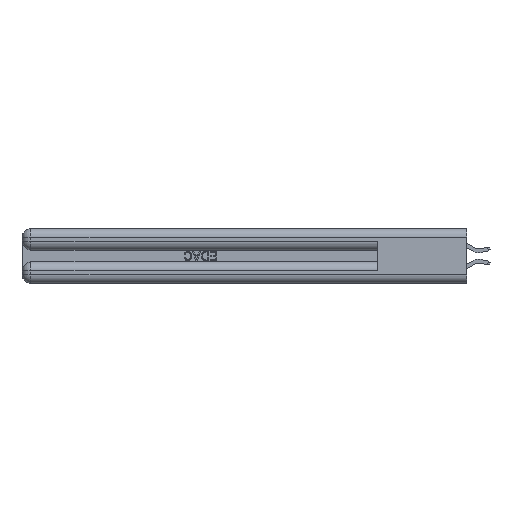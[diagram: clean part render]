
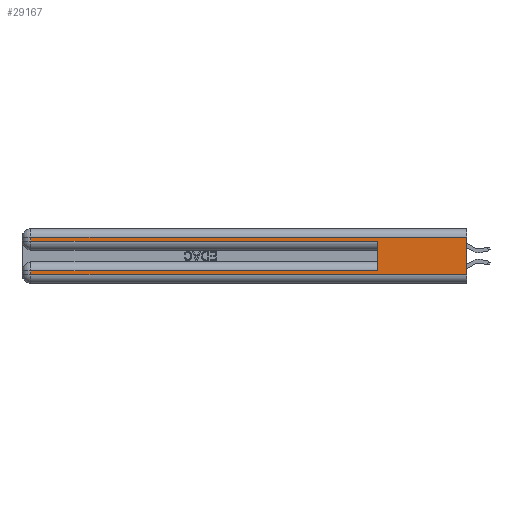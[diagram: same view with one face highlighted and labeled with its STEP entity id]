
A CAD part, left-side view. The second image highlights one B-rep face of the part: STEP entity #29167.
In plain terms, the highlighted planar face has unit normal (-1, 0, 0).
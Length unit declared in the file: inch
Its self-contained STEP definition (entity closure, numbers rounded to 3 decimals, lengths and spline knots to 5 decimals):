
#72 = CARTESIAN_POINT ( 'NONE',  ( 0., 0.6, 0.285 ) ) ;
#311 = EDGE_CURVE ( 'NONE', #539, #42509, #31341, .T. ) ;
#539 = VERTEX_POINT ( 'NONE', #27123 ) ;
#3515 = VERTEX_POINT ( 'NONE', #72 ) ;
#4661 = EDGE_CURVE ( 'NONE', #33282, #26031, #31007, .T. ) ;
#6247 = VERTEX_POINT ( 'NONE', #28322 ) ;
#6253 = CARTESIAN_POINT ( 'NONE',  ( 0., 0., 0.31 ) ) ;
#6600 = DIRECTION ( 'NONE',  ( 0., -1., 0. ) ) ;
#6920 = CARTESIAN_POINT ( 'NONE',  ( 0., 2.94, 0.285 ) ) ;
#7168 = ORIENTED_EDGE ( 'NONE', *, *, #311, .F. ) ;
#7199 = PLANE ( 'NONE',  #31934 ) ;
#7261 = ORIENTED_EDGE ( 'NONE', *, *, #28585, .T. ) ;
#7619 = VECTOR ( 'NONE', #19460, 39.37008 ) ;
#10107 = DIRECTION ( 'NONE',  ( 1., 0., 0. ) ) ;
#10196 = DIRECTION ( 'NONE',  ( 0., 0., -1. ) ) ;
#10818 = CARTESIAN_POINT ( 'NONE',  ( 0., 0.6, 0.145 ) ) ;
#11771 = CARTESIAN_POINT ( 'NONE',  ( 0., 2.94, 0.06 ) ) ;
#12688 = CARTESIAN_POINT ( 'NONE',  ( 0., 0., 0.285 ) ) ;
#13063 = DIRECTION ( 'NONE',  ( 0., 1., 0. ) ) ;
#13878 = EDGE_CURVE ( 'NONE', #539, #33282, #35832, .T. ) ;
#14677 = DIRECTION ( 'NONE',  ( 0., 0., -1. ) ) ;
#15259 = VERTEX_POINT ( 'NONE', #18500 ) ;
#15513 = VERTEX_POINT ( 'NONE', #11771 ) ;
#16956 = ORIENTED_EDGE ( 'NONE', *, *, #28069, .F. ) ;
#18350 = VECTOR ( 'NONE', #36685, 39.37008 ) ;
#18500 = CARTESIAN_POINT ( 'NONE',  ( 0., 2.94, 0.085 ) ) ;
#19460 = DIRECTION ( 'NONE',  ( 0., -1., 0. ) ) ;
#19883 = ORIENTED_EDGE ( 'NONE', *, *, #37157, .T. ) ;
#20031 = ORIENTED_EDGE ( 'NONE', *, *, #35923, .T. ) ;
#21222 = CARTESIAN_POINT ( 'NONE',  ( 0., 0., 0.06 ) ) ;
#22033 = ORIENTED_EDGE ( 'NONE', *, *, #35537, .T. ) ;
#22641 = CARTESIAN_POINT ( 'NONE',  ( 0., 2.94, 0.31 ) ) ;
#22929 = FACE_OUTER_BOUND ( 'NONE', #34871, .T. ) ;
#23273 = DIRECTION ( 'NONE',  ( 0., 0., -1. ) ) ;
#24306 = VECTOR ( 'NONE', #10196, 39.37008 ) ;
#26031 = VERTEX_POINT ( 'NONE', #6920 ) ;
#26415 = CARTESIAN_POINT ( 'NONE',  ( 0., 0., 0.06 ) ) ;
#27123 = CARTESIAN_POINT ( 'NONE',  ( 0., 0., 0.31 ) ) ;
#28069 = EDGE_CURVE ( 'NONE', #6247, #3515, #40621, .T. ) ;
#28322 = CARTESIAN_POINT ( 'NONE',  ( 0., 0.6, 0.085 ) ) ;
#28585 = EDGE_CURVE ( 'NONE', #15513, #42509, #28679, .T. ) ;
#28679 = LINE ( 'NONE', #26415, #36419 ) ;
#28843 = DIRECTION ( 'NONE',  ( 0., 1., 0. ) ) ;
#29167 = ADVANCED_FACE ( 'NONE', ( #22929 ), #7199, .F. ) ;
#30457 = VECTOR ( 'NONE', #13063, 39.37008 ) ;
#31007 = LINE ( 'NONE', #40410, #24306 ) ;
#31341 = LINE ( 'NONE', #39829, #42304 ) ;
#31934 = AXIS2_PLACEMENT_3D ( 'NONE', #36413, #10107, #23273 ) ;
#33036 = LINE ( 'NONE', #36187, #30457 ) ;
#33282 = VERTEX_POINT ( 'NONE', #22641 ) ;
#34259 = DIRECTION ( 'NONE',  ( 0., 0., -1. ) ) ;
#34871 = EDGE_LOOP ( 'NONE', ( #7168, #38168, #40610, #19883, #16956, #20031, #22033, #7261 ) ) ;
#35537 = EDGE_CURVE ( 'NONE', #15259, #15513, #39340, .T. ) ;
#35832 = LINE ( 'NONE', #6253, #41044 ) ;
#35923 = EDGE_CURVE ( 'NONE', #6247, #15259, #33036, .T. ) ;
#36187 = CARTESIAN_POINT ( 'NONE',  ( 0., 0., 0.085 ) ) ;
#36413 = CARTESIAN_POINT ( 'NONE',  ( 0., 0., 0.37 ) ) ;
#36419 = VECTOR ( 'NONE', #6600, 39.37008 ) ;
#36685 = DIRECTION ( 'NONE',  ( 0., 0., 1. ) ) ;
#37157 = EDGE_CURVE ( 'NONE', #26031, #3515, #42897, .T. ) ;
#38168 = ORIENTED_EDGE ( 'NONE', *, *, #13878, .T. ) ;
#38277 = VECTOR ( 'NONE', #14677, 39.37008 ) ;
#39340 = LINE ( 'NONE', #40866, #38277 ) ;
#39829 = CARTESIAN_POINT ( 'NONE',  ( 0., 0., 0.37 ) ) ;
#40410 = CARTESIAN_POINT ( 'NONE',  ( 0., 2.94, 0.37 ) ) ;
#40610 = ORIENTED_EDGE ( 'NONE', *, *, #4661, .T. ) ;
#40621 = LINE ( 'NONE', #10818, #18350 ) ;
#40866 = CARTESIAN_POINT ( 'NONE',  ( 0., 2.94, 0.37 ) ) ;
#41044 = VECTOR ( 'NONE', #28843, 39.37008 ) ;
#42304 = VECTOR ( 'NONE', #34259, 39.37008 ) ;
#42509 = VERTEX_POINT ( 'NONE', #21222 ) ;
#42897 = LINE ( 'NONE', #12688, #7619 ) ;
